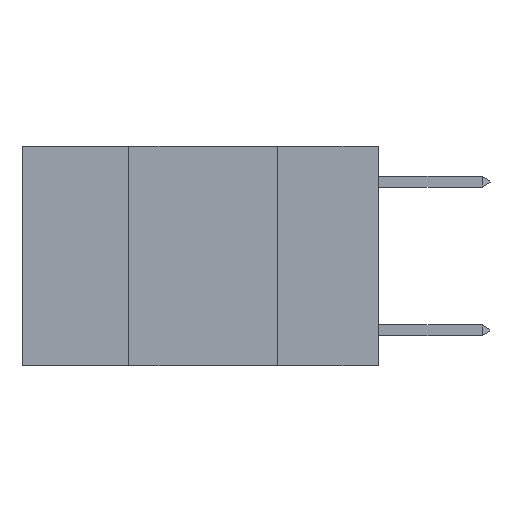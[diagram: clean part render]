
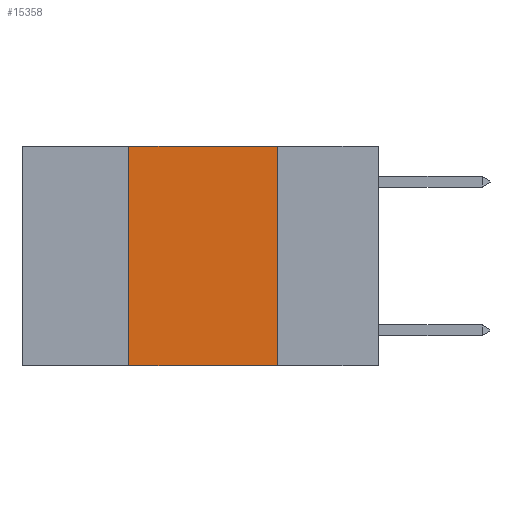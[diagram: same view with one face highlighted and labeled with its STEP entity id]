
A CAD part, left-side view. The second image highlights one B-rep face of the part: STEP entity #15358.
In plain terms, the highlighted planar face has unit normal (-1, 0, 0).
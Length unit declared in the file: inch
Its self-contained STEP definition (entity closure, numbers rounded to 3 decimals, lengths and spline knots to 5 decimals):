
#1650 = ORIENTED_EDGE ( 'NONE', *, *, #8972, .T. ) ;
#3348 = EDGE_CURVE ( 'NONE', #17218, #17412, #18555, .T. ) ;
#5244 = LINE ( 'NONE', #12983, #24073 ) ;
#5577 = CARTESIAN_POINT ( 'NONE',  ( 0., 0.42, -0.37 ) ) ;
#5697 = CARTESIAN_POINT ( 'NONE',  ( 0., 0.17, -0.37 ) ) ;
#7526 = EDGE_LOOP ( 'NONE', ( #17673, #14997, #22893, #1650 ) ) ;
#7714 = CARTESIAN_POINT ( 'NONE',  ( 0., 0.6, 0. ) ) ;
#7823 = LINE ( 'NONE', #29952, #18425 ) ;
#8095 = DIRECTION ( 'NONE',  ( 0., 0., -1. ) ) ;
#8592 = CARTESIAN_POINT ( 'NONE',  ( 0., 0.6, 0. ) ) ;
#8972 = EDGE_CURVE ( 'NONE', #23099, #17614, #7823, .T. ) ;
#10083 = FACE_OUTER_BOUND ( 'NONE', #7526, .T. ) ;
#10510 = CARTESIAN_POINT ( 'NONE',  ( 0., 0.42, 0. ) ) ;
#11560 = AXIS2_PLACEMENT_3D ( 'NONE', #7714, #17359, #25410 ) ;
#12983 = CARTESIAN_POINT ( 'NONE',  ( 0., 0.17, 0. ) ) ;
#14660 = CARTESIAN_POINT ( 'NONE',  ( 0., 0.42, 0. ) ) ;
#14997 = ORIENTED_EDGE ( 'NONE', *, *, #3348, .F. ) ;
#15358 = ADVANCED_FACE ( 'NONE', ( #10083 ), #19732, .F. ) ;
#16549 = EDGE_CURVE ( 'NONE', #23099, #17218, #21795, .T. ) ;
#17036 = VECTOR ( 'NONE', #20772, 39.37008 ) ;
#17218 = VERTEX_POINT ( 'NONE', #10510 ) ;
#17359 = DIRECTION ( 'NONE',  ( 1., 0., 0. ) ) ;
#17412 = VERTEX_POINT ( 'NONE', #26306 ) ;
#17614 = VERTEX_POINT ( 'NONE', #5697 ) ;
#17673 = ORIENTED_EDGE ( 'NONE', *, *, #25005, .F. ) ;
#18425 = VECTOR ( 'NONE', #24747, 39.37008 ) ;
#18555 = LINE ( 'NONE', #8592, #17036 ) ;
#19732 = PLANE ( 'NONE',  #11560 ) ;
#20772 = DIRECTION ( 'NONE',  ( 0., -1., 0. ) ) ;
#21795 = LINE ( 'NONE', #14660, #22759 ) ;
#22759 = VECTOR ( 'NONE', #28904, 39.37008 ) ;
#22893 = ORIENTED_EDGE ( 'NONE', *, *, #16549, .F. ) ;
#23099 = VERTEX_POINT ( 'NONE', #5577 ) ;
#24073 = VECTOR ( 'NONE', #8095, 39.37008 ) ;
#24747 = DIRECTION ( 'NONE',  ( 0., -1., 0. ) ) ;
#25005 = EDGE_CURVE ( 'NONE', #17412, #17614, #5244, .T. ) ;
#25410 = DIRECTION ( 'NONE',  ( 0., 0., -1. ) ) ;
#26306 = CARTESIAN_POINT ( 'NONE',  ( 0., 0.17, 0. ) ) ;
#28904 = DIRECTION ( 'NONE',  ( 0., 0., 1. ) ) ;
#29952 = CARTESIAN_POINT ( 'NONE',  ( 0., 0.6, -0.37 ) ) ;
